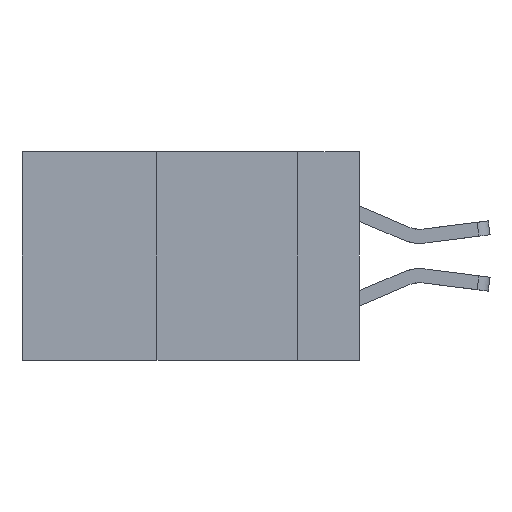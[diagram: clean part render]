
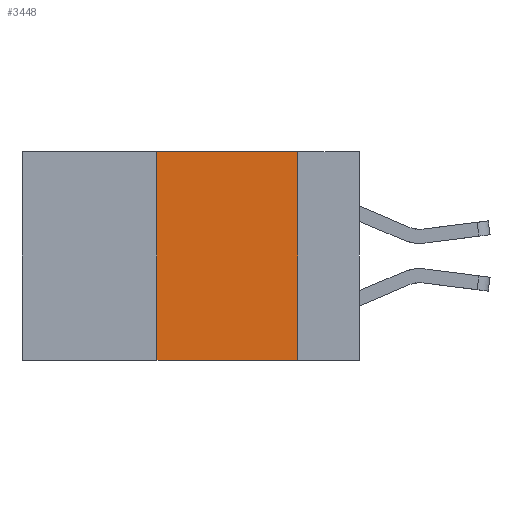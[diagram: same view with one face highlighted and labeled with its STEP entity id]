
A CAD part, left-side view. The second image highlights one B-rep face of the part: STEP entity #3448.
In plain terms, the highlighted planar face has unit normal (-1, 0, 0).
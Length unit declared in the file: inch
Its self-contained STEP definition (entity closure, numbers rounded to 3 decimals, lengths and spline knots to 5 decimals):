
#585 = FACE_OUTER_BOUND ( 'NONE', #8206, .T. ) ;
#986 = VERTEX_POINT ( 'NONE', #8549 ) ;
#1595 = DIRECTION ( 'NONE',  ( 0., -1., 0. ) ) ;
#1943 = ORIENTED_EDGE ( 'NONE', *, *, #2400, .F. ) ;
#2400 = EDGE_CURVE ( 'NONE', #13986, #12118, #4591, .T. ) ;
#3169 = PLANE ( 'NONE',  #14264 ) ;
#3258 = CARTESIAN_POINT ( 'NONE',  ( 0., 0.6, 0. ) ) ;
#3448 = ADVANCED_FACE ( 'NONE', ( #585 ), #3169, .F. ) ;
#4081 = CARTESIAN_POINT ( 'NONE',  ( 0., 0.36, 0. ) ) ;
#4591 = LINE ( 'NONE', #6980, #13015 ) ;
#4769 = DIRECTION ( 'NONE',  ( 0., 0., -1. ) ) ;
#5088 = CARTESIAN_POINT ( 'NONE',  ( 0., 0.11, 0. ) ) ;
#5353 = DIRECTION ( 'NONE',  ( 1., 0., 0. ) ) ;
#5539 = VECTOR ( 'NONE', #9045, 39.37008 ) ;
#5680 = CARTESIAN_POINT ( 'NONE',  ( 0., 0.6, 0. ) ) ;
#5710 = LINE ( 'NONE', #5680, #5539 ) ;
#6354 = ORIENTED_EDGE ( 'NONE', *, *, #12814, .F. ) ;
#6429 = LINE ( 'NONE', #13993, #10100 ) ;
#6980 = CARTESIAN_POINT ( 'NONE',  ( 0., 0.11, 0. ) ) ;
#7437 = VERTEX_POINT ( 'NONE', #4081 ) ;
#7582 = ORIENTED_EDGE ( 'NONE', *, *, #8643, .F. ) ;
#8206 = EDGE_LOOP ( 'NONE', ( #1943, #7582, #6354, #9450 ) ) ;
#8549 = CARTESIAN_POINT ( 'NONE',  ( 0., 0.36, -0.37 ) ) ;
#8643 = EDGE_CURVE ( 'NONE', #7437, #13986, #5710, .T. ) ;
#9026 = LINE ( 'NONE', #10529, #11819 ) ;
#9045 = DIRECTION ( 'NONE',  ( 0., -1., 0. ) ) ;
#9450 = ORIENTED_EDGE ( 'NONE', *, *, #13847, .T. ) ;
#10005 = CARTESIAN_POINT ( 'NONE',  ( 0., 0.11, -0.37 ) ) ;
#10100 = VECTOR ( 'NONE', #11781, 39.37008 ) ;
#10529 = CARTESIAN_POINT ( 'NONE',  ( 0., 0.6, -0.37 ) ) ;
#11781 = DIRECTION ( 'NONE',  ( 0., 0., 1. ) ) ;
#11819 = VECTOR ( 'NONE', #1595, 39.37008 ) ;
#12118 = VERTEX_POINT ( 'NONE', #10005 ) ;
#12814 = EDGE_CURVE ( 'NONE', #986, #7437, #6429, .T. ) ;
#13015 = VECTOR ( 'NONE', #4769, 39.37008 ) ;
#13318 = DIRECTION ( 'NONE',  ( 0., 0., -1. ) ) ;
#13847 = EDGE_CURVE ( 'NONE', #986, #12118, #9026, .T. ) ;
#13986 = VERTEX_POINT ( 'NONE', #5088 ) ;
#13993 = CARTESIAN_POINT ( 'NONE',  ( 0., 0.36, 0. ) ) ;
#14264 = AXIS2_PLACEMENT_3D ( 'NONE', #3258, #5353, #13318 ) ;
